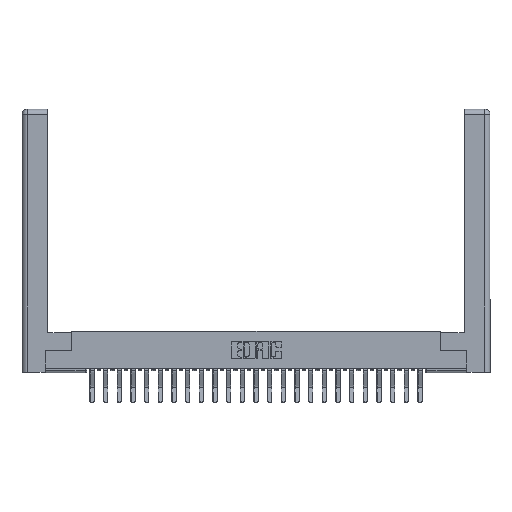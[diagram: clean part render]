
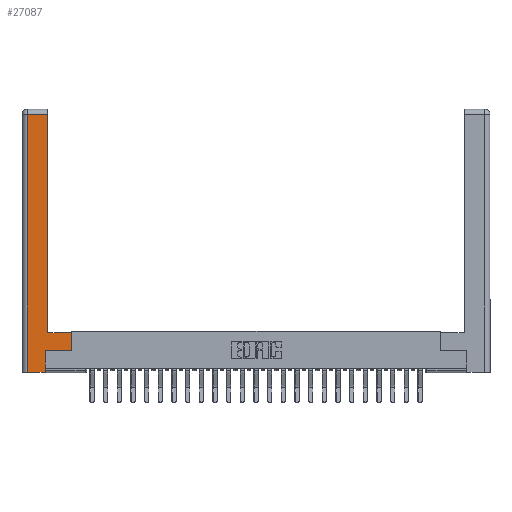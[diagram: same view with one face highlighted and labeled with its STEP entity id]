
A CAD part, top view. The second image highlights one B-rep face of the part: STEP entity #27087.
In plain terms, the highlighted planar face has unit normal (0, 0, 1).
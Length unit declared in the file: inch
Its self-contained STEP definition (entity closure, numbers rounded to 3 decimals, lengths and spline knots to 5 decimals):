
#126 = LINE ( 'NONE', #10795, #15505 ) ;
#1195 = LINE ( 'NONE', #22258, #10999 ) ;
#1225 = DIRECTION ( 'NONE',  ( 1., 0., 0. ) ) ;
#1284 = VERTEX_POINT ( 'NONE', #23006 ) ;
#1332 = CARTESIAN_POINT ( 'NONE',  ( 0.295, 2.94, 0. ) ) ;
#1342 = CARTESIAN_POINT ( 'NONE',  ( 0.265, 0.245, 0. ) ) ;
#1471 = ORIENTED_EDGE ( 'NONE', *, *, #8653, .T. ) ;
#1493 = EDGE_CURVE ( 'NONE', #14614, #4304, #20472, .T. ) ;
#1745 = CARTESIAN_POINT ( 'NONE',  ( 0.0615, 0., 0. ) ) ;
#2238 = ORIENTED_EDGE ( 'NONE', *, *, #4173, .T. ) ;
#2360 = PLANE ( 'NONE',  #26750 ) ;
#2874 = EDGE_CURVE ( 'NONE', #1284, #14614, #11162, .T. ) ;
#3792 = EDGE_CURVE ( 'NONE', #6613, #1284, #7143, .T. ) ;
#4173 = EDGE_CURVE ( 'NONE', #4304, #19410, #11083, .T. ) ;
#4239 = CARTESIAN_POINT ( 'NONE',  ( 0.565, 0.45, 0. ) ) ;
#4304 = VERTEX_POINT ( 'NONE', #21704 ) ;
#4408 = DIRECTION ( 'NONE',  ( 0., 1., 0. ) ) ;
#4689 = EDGE_LOOP ( 'NONE', ( #1471, #24799, #10418, #13756, #23129, #14094, #26145, #2238 ) ) ;
#6342 = EDGE_CURVE ( 'NONE', #8237, #6613, #1195, .T. ) ;
#6357 = CARTESIAN_POINT ( 'NONE',  ( 0.295, 0.45, 0. ) ) ;
#6383 = DIRECTION ( 'NONE',  ( 0., -1., 0. ) ) ;
#6613 = VERTEX_POINT ( 'NONE', #18676 ) ;
#6642 = DIRECTION ( 'NONE',  ( -1., 0., 0. ) ) ;
#7143 = LINE ( 'NONE', #1342, #21894 ) ;
#8237 = VERTEX_POINT ( 'NONE', #1745 ) ;
#8653 = EDGE_CURVE ( 'NONE', #19410, #22545, #26583, .T. ) ;
#9944 = CARTESIAN_POINT ( 'NONE',  ( 0.565, 0.245, 0. ) ) ;
#10418 = ORIENTED_EDGE ( 'NONE', *, *, #11088, .T. ) ;
#10795 = CARTESIAN_POINT ( 'NONE',  ( 0.0615, 0., 0. ) ) ;
#10963 = EDGE_CURVE ( 'NONE', #22545, #18633, #11257, .T. ) ;
#10991 = CARTESIAN_POINT ( 'NONE',  ( 0.295, 0.45, 0. ) ) ;
#10999 = VECTOR ( 'NONE', #1225, 39.37008 ) ;
#11083 = LINE ( 'NONE', #10991, #17949 ) ;
#11088 = EDGE_CURVE ( 'NONE', #18633, #8237, #126, .T. ) ;
#11162 = LINE ( 'NONE', #9944, #16049 ) ;
#11254 = DIRECTION ( 'NONE',  ( 0., 1., 0. ) ) ;
#11257 = LINE ( 'NONE', #12354, #21730 ) ;
#12354 = CARTESIAN_POINT ( 'NONE',  ( 0.0615, 2.94, 0. ) ) ;
#12480 = CARTESIAN_POINT ( 'NONE',  ( 0.565, 0.245, 0. ) ) ;
#12890 = DIRECTION ( 'NONE',  ( -1., 0., 0. ) ) ;
#13756 = ORIENTED_EDGE ( 'NONE', *, *, #6342, .T. ) ;
#13822 = VECTOR ( 'NONE', #11254, 39.37008 ) ;
#14094 = ORIENTED_EDGE ( 'NONE', *, *, #2874, .T. ) ;
#14614 = VERTEX_POINT ( 'NONE', #12480 ) ;
#15505 = VECTOR ( 'NONE', #6383, 39.37008 ) ;
#16049 = VECTOR ( 'NONE', #18233, 39.37008 ) ;
#17949 = VECTOR ( 'NONE', #12890, 39.37008 ) ;
#17968 = DIRECTION ( 'NONE',  ( 0., 1., 0. ) ) ;
#18233 = DIRECTION ( 'NONE',  ( 1., 0., 0. ) ) ;
#18484 = DIRECTION ( 'NONE',  ( -1., 0., 0. ) ) ;
#18633 = VERTEX_POINT ( 'NONE', #24444 ) ;
#18676 = CARTESIAN_POINT ( 'NONE',  ( 0.265, 0., 0. ) ) ;
#19389 = CARTESIAN_POINT ( 'NONE',  ( 0., 0., 0. ) ) ;
#19410 = VERTEX_POINT ( 'NONE', #6357 ) ;
#20472 = LINE ( 'NONE', #4239, #26013 ) ;
#21704 = CARTESIAN_POINT ( 'NONE',  ( 0.565, 0.45, 0. ) ) ;
#21730 = VECTOR ( 'NONE', #18484, 39.37008 ) ;
#21894 = VECTOR ( 'NONE', #17968, 39.37008 ) ;
#22044 = CARTESIAN_POINT ( 'NONE',  ( 0.295, 3., 0. ) ) ;
#22258 = CARTESIAN_POINT ( 'NONE',  ( 0.265, 0., 0. ) ) ;
#22545 = VERTEX_POINT ( 'NONE', #1332 ) ;
#23006 = CARTESIAN_POINT ( 'NONE',  ( 0.265, 0.245, 0. ) ) ;
#23129 = ORIENTED_EDGE ( 'NONE', *, *, #3792, .T. ) ;
#24444 = CARTESIAN_POINT ( 'NONE',  ( 0.0615, 2.94, 0. ) ) ;
#24799 = ORIENTED_EDGE ( 'NONE', *, *, #10963, .T. ) ;
#25325 = DIRECTION ( 'NONE',  ( 0., 0., -1. ) ) ;
#25601 = FACE_OUTER_BOUND ( 'NONE', #4689, .T. ) ;
#26013 = VECTOR ( 'NONE', #4408, 39.37008 ) ;
#26145 = ORIENTED_EDGE ( 'NONE', *, *, #1493, .T. ) ;
#26583 = LINE ( 'NONE', #22044, #13822 ) ;
#26750 = AXIS2_PLACEMENT_3D ( 'NONE', #19389, #25325, #6642 ) ;
#27087 = ADVANCED_FACE ( 'NONE', ( #25601 ), #2360, .F. ) ;
